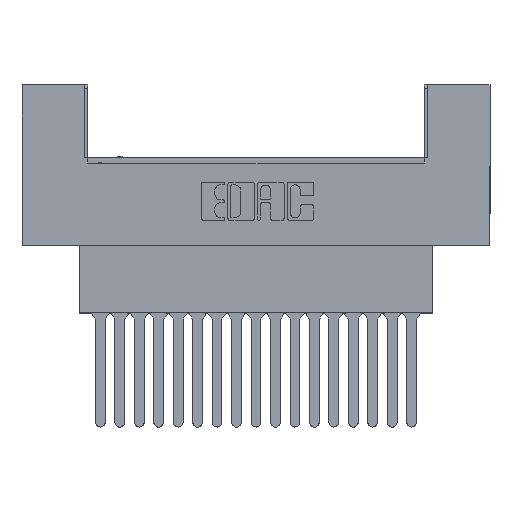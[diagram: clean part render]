
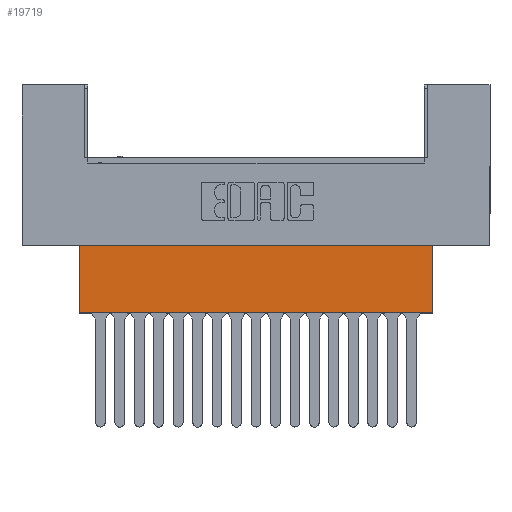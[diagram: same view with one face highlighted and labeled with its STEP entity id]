
A CAD part, top view. The second image highlights one B-rep face of the part: STEP entity #19719.
In plain terms, the highlighted planar face has unit normal (0, 0, 1).
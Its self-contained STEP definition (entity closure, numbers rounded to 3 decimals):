
#379 = CARTESIAN_POINT ( 'NONE',  ( 7.468, -8.814, -3.962 ) ) ;
#478 = CARTESIAN_POINT ( 'NONE',  ( 53.645, -8.814, -3.962 ) ) ;
#1116 = LINE ( 'NONE', #6143, #22865 ) ;
#2668 = AXIS2_PLACEMENT_3D ( 'NONE', #20630, #11142, #5617 ) ;
#3236 = EDGE_CURVE ( 'NONE', #10384, #22928, #1116, .T. ) ;
#3533 = EDGE_CURVE ( 'NONE', #22928, #20157, #22245, .T. ) ;
#3805 = EDGE_CURVE ( 'NONE', #22592, #20157, #8735, .T. ) ;
#5160 = EDGE_LOOP ( 'NONE', ( #20556, #14288, #15022, #21656 ) ) ;
#5617 = DIRECTION ( 'NONE',  ( 0., 1., 0. ) ) ;
#6143 = CARTESIAN_POINT ( 'NONE',  ( 61.112, -8.814, -3.962 ) ) ;
#6238 = EDGE_CURVE ( 'NONE', #22592, #10384, #20050, .T. ) ;
#7756 = VECTOR ( 'NONE', #20472, 1000. ) ;
#8267 = DIRECTION ( 'NONE',  ( -1., 0., 0. ) ) ;
#8735 = LINE ( 'NONE', #17811, #12508 ) ;
#9142 = CARTESIAN_POINT ( 'NONE',  ( 53.645, 0., -3.962 ) ) ;
#10384 = VERTEX_POINT ( 'NONE', #478 ) ;
#11142 = DIRECTION ( 'NONE',  ( 0., 0., -1. ) ) ;
#11272 = FACE_OUTER_BOUND ( 'NONE', #5160, .T. ) ;
#11338 = VECTOR ( 'NONE', #19104, 1000. ) ;
#12508 = VECTOR ( 'NONE', #19587, 1000. ) ;
#13106 = PLANE ( 'NONE',  #2668 ) ;
#13406 = CARTESIAN_POINT ( 'NONE',  ( 7.468, 0., -3.962 ) ) ;
#14288 = ORIENTED_EDGE ( 'NONE', *, *, #6238, .F. ) ;
#15022 = ORIENTED_EDGE ( 'NONE', *, *, #3805, .T. ) ;
#16747 = CARTESIAN_POINT ( 'NONE',  ( 53.645, -8.814, -3.962 ) ) ;
#17811 = CARTESIAN_POINT ( 'NONE',  ( 61.112, 0., -3.962 ) ) ;
#19104 = DIRECTION ( 'NONE',  ( 0., 1., 0. ) ) ;
#19587 = DIRECTION ( 'NONE',  ( -1., 0., 0. ) ) ;
#19719 = ADVANCED_FACE ( 'NONE', ( #11272 ), #13106, .F. ) ;
#20050 = LINE ( 'NONE', #16747, #7756 ) ;
#20157 = VERTEX_POINT ( 'NONE', #13406 ) ;
#20472 = DIRECTION ( 'NONE',  ( 0., -1., 0. ) ) ;
#20556 = ORIENTED_EDGE ( 'NONE', *, *, #3236, .F. ) ;
#20630 = CARTESIAN_POINT ( 'NONE',  ( 61.112, 0., -3.962 ) ) ;
#21656 = ORIENTED_EDGE ( 'NONE', *, *, #3533, .F. ) ;
#22245 = LINE ( 'NONE', #22838, #11338 ) ;
#22592 = VERTEX_POINT ( 'NONE', #9142 ) ;
#22838 = CARTESIAN_POINT ( 'NONE',  ( 7.468, -8.814, -3.962 ) ) ;
#22865 = VECTOR ( 'NONE', #8267, 1000. ) ;
#22928 = VERTEX_POINT ( 'NONE', #379 ) ;
